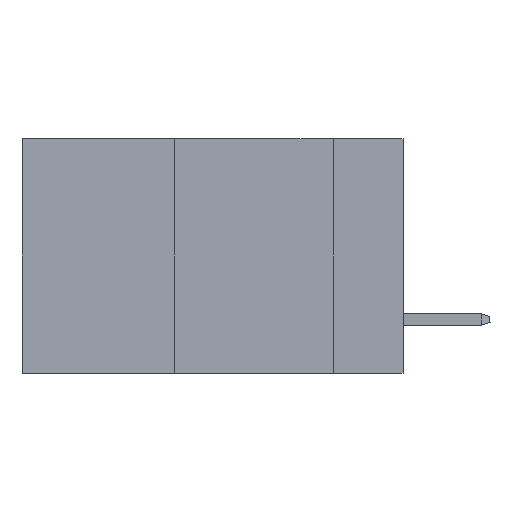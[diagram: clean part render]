
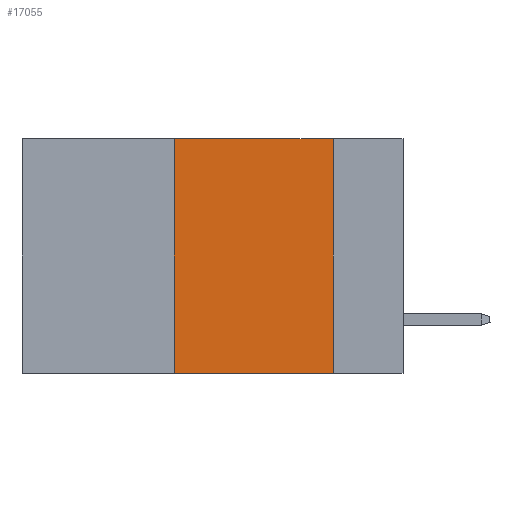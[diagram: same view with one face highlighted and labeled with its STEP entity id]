
A CAD part, left-side view. The second image highlights one B-rep face of the part: STEP entity #17055.
In plain terms, the highlighted planar face has unit normal (-1, 0, 0).
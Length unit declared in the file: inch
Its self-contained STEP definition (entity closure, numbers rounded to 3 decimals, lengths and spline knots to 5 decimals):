
#3658 = ORIENTED_EDGE ( 'NONE', *, *, #25382, .F. ) ;
#5577 = ORIENTED_EDGE ( 'NONE', *, *, #34658, .F. ) ;
#6736 = DIRECTION ( 'NONE',  ( 0., -1., 0. ) ) ;
#7203 = ORIENTED_EDGE ( 'NONE', *, *, #35659, .F. ) ;
#7538 = EDGE_LOOP ( 'NONE', ( #7203, #5577, #3658, #24531 ) ) ;
#10817 = CARTESIAN_POINT ( 'NONE',  ( 0., 0.36, 0. ) ) ;
#11070 = VECTOR ( 'NONE', #41849, 39.37008 ) ;
#13192 = CARTESIAN_POINT ( 'NONE',  ( 0., 0.6, -0.37 ) ) ;
#14236 = CARTESIAN_POINT ( 'NONE',  ( 0., 0.36, -0.37 ) ) ;
#14512 = LINE ( 'NONE', #37929, #11070 ) ;
#15359 = LINE ( 'NONE', #25895, #25724 ) ;
#15989 = VERTEX_POINT ( 'NONE', #42171 ) ;
#17055 = ADVANCED_FACE ( 'NONE', ( #33309 ), #26903, .F. ) ;
#18757 = VERTEX_POINT ( 'NONE', #14236 ) ;
#20019 = DIRECTION ( 'NONE',  ( 0., 0., -1. ) ) ;
#22398 = VECTOR ( 'NONE', #30833, 39.37008 ) ;
#23474 = CARTESIAN_POINT ( 'NONE',  ( 0., 0.6, 0. ) ) ;
#24531 = ORIENTED_EDGE ( 'NONE', *, *, #39451, .T. ) ;
#25382 = EDGE_CURVE ( 'NONE', #18757, #39602, #27619, .T. ) ;
#25724 = VECTOR ( 'NONE', #27496, 39.37008 ) ;
#25743 = AXIS2_PLACEMENT_3D ( 'NONE', #23474, #44166, #20019 ) ;
#25895 = CARTESIAN_POINT ( 'NONE',  ( 0., 0.6, 0. ) ) ;
#26903 = PLANE ( 'NONE',  #25743 ) ;
#27496 = DIRECTION ( 'NONE',  ( 0., -1., 0. ) ) ;
#27619 = LINE ( 'NONE', #10817, #22398 ) ;
#28299 = CARTESIAN_POINT ( 'NONE',  ( 0., 0.36, 0. ) ) ;
#29427 = VECTOR ( 'NONE', #6736, 39.37008 ) ;
#30280 = CARTESIAN_POINT ( 'NONE',  ( 0., 0.11, 0. ) ) ;
#30833 = DIRECTION ( 'NONE',  ( 0., 0., 1. ) ) ;
#33309 = FACE_OUTER_BOUND ( 'NONE', #7538, .T. ) ;
#34658 = EDGE_CURVE ( 'NONE', #39602, #43453, #15359, .T. ) ;
#35659 = EDGE_CURVE ( 'NONE', #43453, #15989, #14512, .T. ) ;
#37733 = LINE ( 'NONE', #13192, #29427 ) ;
#37929 = CARTESIAN_POINT ( 'NONE',  ( 0., 0.11, 0. ) ) ;
#39451 = EDGE_CURVE ( 'NONE', #18757, #15989, #37733, .T. ) ;
#39602 = VERTEX_POINT ( 'NONE', #28299 ) ;
#41849 = DIRECTION ( 'NONE',  ( 0., 0., -1. ) ) ;
#42171 = CARTESIAN_POINT ( 'NONE',  ( 0., 0.11, -0.37 ) ) ;
#43453 = VERTEX_POINT ( 'NONE', #30280 ) ;
#44166 = DIRECTION ( 'NONE',  ( 1., 0., 0. ) ) ;
